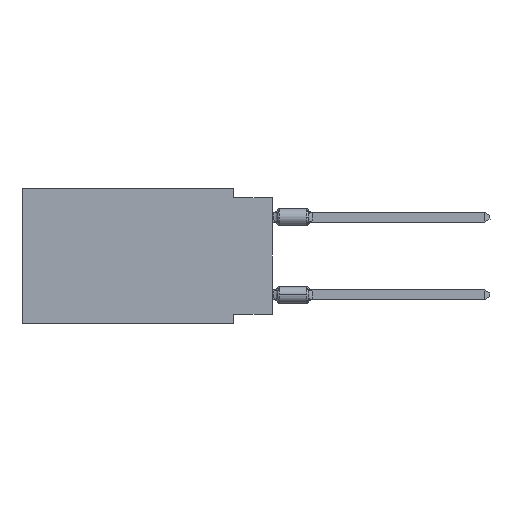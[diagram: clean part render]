
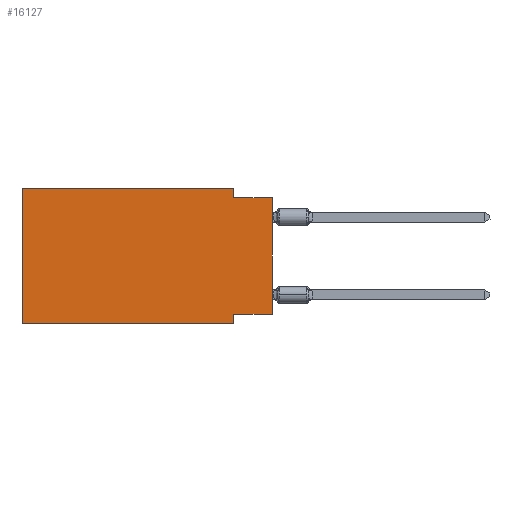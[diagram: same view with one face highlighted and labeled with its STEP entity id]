
A CAD part, left-side view. The second image highlights one B-rep face of the part: STEP entity #16127.
In plain terms, the highlighted planar face has unit normal (-1, 0, 0).
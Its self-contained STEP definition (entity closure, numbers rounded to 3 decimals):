
#236 = EDGE_CURVE ( 'NONE', #4896, #648, #3799, .T. ) ;
#472 = DIRECTION ( 'NONE',  ( 0., -1., 0. ) ) ;
#648 = VERTEX_POINT ( 'NONE', #3615 ) ;
#1191 = CARTESIAN_POINT ( 'NONE',  ( 0., 0., -8.255 ) ) ;
#1465 = ORIENTED_EDGE ( 'NONE', *, *, #1579, .F. ) ;
#1579 = EDGE_CURVE ( 'NONE', #4043, #7565, #5329, .T. ) ;
#1584 = EDGE_CURVE ( 'NONE', #16424, #4043, #2900, .T. ) ;
#2359 = EDGE_CURVE ( 'NONE', #648, #10372, #5986, .T. ) ;
#2385 = CARTESIAN_POINT ( 'NONE',  ( 0., 0., -0.635 ) ) ;
#2718 = CARTESIAN_POINT ( 'NONE',  ( 0., 2.54, -0.635 ) ) ;
#2824 = VECTOR ( 'NONE', #6665, 1000. ) ;
#2900 = LINE ( 'NONE', #7680, #6897 ) ;
#3490 = EDGE_CURVE ( 'NONE', #4896, #7565, #11756, .T. ) ;
#3615 = CARTESIAN_POINT ( 'NONE',  ( 0., 2.54, -8.255 ) ) ;
#3799 = LINE ( 'NONE', #1191, #9059 ) ;
#3855 = LINE ( 'NONE', #14061, #9758 ) ;
#3865 = VECTOR ( 'NONE', #8425, 1000. ) ;
#4043 = VERTEX_POINT ( 'NONE', #2718 ) ;
#4074 = DIRECTION ( 'NONE',  ( 0., -1., 0. ) ) ;
#4322 = ORIENTED_EDGE ( 'NONE', *, *, #236, .F. ) ;
#4896 = VERTEX_POINT ( 'NONE', #16196 ) ;
#5329 = LINE ( 'NONE', #9013, #10104 ) ;
#5627 = FACE_OUTER_BOUND ( 'NONE', #9619, .T. ) ;
#5986 = LINE ( 'NONE', #12270, #3865 ) ;
#6030 = CARTESIAN_POINT ( 'NONE',  ( 0., 16.383, 0. ) ) ;
#6135 = EDGE_CURVE ( 'NONE', #8010, #16424, #14717, .T. ) ;
#6298 = DIRECTION ( 'NONE',  ( 0., 1., 0. ) ) ;
#6510 = ORIENTED_EDGE ( 'NONE', *, *, #1584, .F. ) ;
#6665 = DIRECTION ( 'NONE',  ( 0., 0., 1. ) ) ;
#6726 = DIRECTION ( 'NONE',  ( 0., -1., 0. ) ) ;
#6800 = LINE ( 'NONE', #7746, #15700 ) ;
#6897 = VECTOR ( 'NONE', #14280, 1000. ) ;
#7565 = VERTEX_POINT ( 'NONE', #2385 ) ;
#7680 = CARTESIAN_POINT ( 'NONE',  ( 0., 2.54, 0. ) ) ;
#7746 = CARTESIAN_POINT ( 'NONE',  ( 0., 16.383, -8.89 ) ) ;
#8010 = VERTEX_POINT ( 'NONE', #12565 ) ;
#8063 = EDGE_CURVE ( 'NONE', #9588, #8010, #3855, .T. ) ;
#8220 = AXIS2_PLACEMENT_3D ( 'NONE', #6030, #9800, #15004 ) ;
#8425 = DIRECTION ( 'NONE',  ( 0., 0., -1. ) ) ;
#9013 = CARTESIAN_POINT ( 'NONE',  ( 0., 0., -0.635 ) ) ;
#9059 = VECTOR ( 'NONE', #6298, 1000. ) ;
#9225 = ORIENTED_EDGE ( 'NONE', *, *, #8063, .F. ) ;
#9363 = CARTESIAN_POINT ( 'NONE',  ( 0., 16.383, 0. ) ) ;
#9588 = VERTEX_POINT ( 'NONE', #12786 ) ;
#9619 = EDGE_LOOP ( 'NONE', ( #14721, #1465, #6510, #12930, #9225, #16344, #12035, #4322 ) ) ;
#9758 = VECTOR ( 'NONE', #15326, 1000. ) ;
#9800 = DIRECTION ( 'NONE',  ( 1., 0., 0. ) ) ;
#10104 = VECTOR ( 'NONE', #4074, 1000. ) ;
#10357 = VECTOR ( 'NONE', #472, 1000. ) ;
#10372 = VERTEX_POINT ( 'NONE', #10714 ) ;
#10714 = CARTESIAN_POINT ( 'NONE',  ( 0., 2.54, -8.89 ) ) ;
#11756 = LINE ( 'NONE', #12921, #2824 ) ;
#12035 = ORIENTED_EDGE ( 'NONE', *, *, #2359, .F. ) ;
#12270 = CARTESIAN_POINT ( 'NONE',  ( 0., 2.54, -8.89 ) ) ;
#12565 = CARTESIAN_POINT ( 'NONE',  ( 0., 16.383, 0. ) ) ;
#12786 = CARTESIAN_POINT ( 'NONE',  ( 0., 16.383, -8.89 ) ) ;
#12921 = CARTESIAN_POINT ( 'NONE',  ( 0., 0., 0. ) ) ;
#12930 = ORIENTED_EDGE ( 'NONE', *, *, #6135, .F. ) ;
#13322 = PLANE ( 'NONE',  #8220 ) ;
#14061 = CARTESIAN_POINT ( 'NONE',  ( 0., 16.383, 0. ) ) ;
#14280 = DIRECTION ( 'NONE',  ( 0., 0., -1. ) ) ;
#14560 = CARTESIAN_POINT ( 'NONE',  ( 0., 2.54, 0. ) ) ;
#14717 = LINE ( 'NONE', #9363, #10357 ) ;
#14721 = ORIENTED_EDGE ( 'NONE', *, *, #3490, .T. ) ;
#15004 = DIRECTION ( 'NONE',  ( 0., 0., -1. ) ) ;
#15326 = DIRECTION ( 'NONE',  ( 0., 0., 1. ) ) ;
#15700 = VECTOR ( 'NONE', #6726, 1000. ) ;
#15981 = EDGE_CURVE ( 'NONE', #9588, #10372, #6800, .T. ) ;
#16127 = ADVANCED_FACE ( 'NONE', ( #5627 ), #13322, .F. ) ;
#16196 = CARTESIAN_POINT ( 'NONE',  ( 0., 0., -8.255 ) ) ;
#16344 = ORIENTED_EDGE ( 'NONE', *, *, #15981, .T. ) ;
#16424 = VERTEX_POINT ( 'NONE', #14560 ) ;
